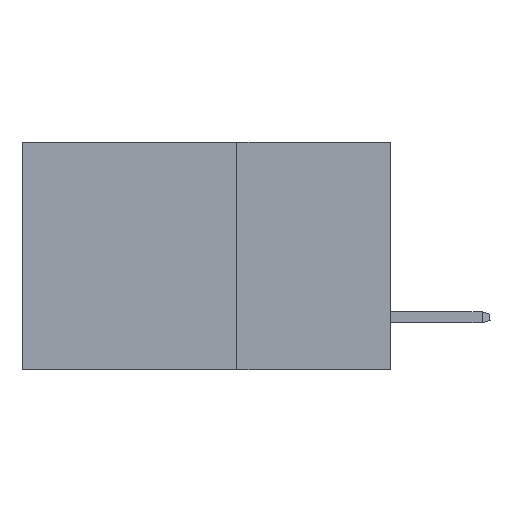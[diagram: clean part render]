
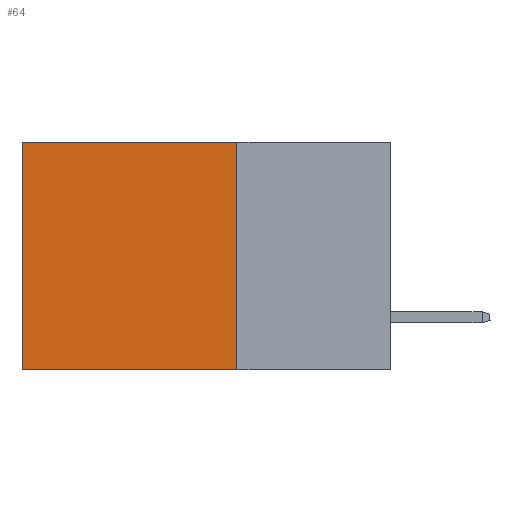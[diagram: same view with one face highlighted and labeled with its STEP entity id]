
A CAD part, left-side view. The second image highlights one B-rep face of the part: STEP entity #64.
In plain terms, the highlighted planar face has unit normal (-1, 0, 0).
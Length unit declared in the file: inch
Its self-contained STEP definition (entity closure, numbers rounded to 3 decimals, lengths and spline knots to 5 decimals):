
#64 = ADVANCED_FACE ( 'NONE', ( #3628 ), #10344, .F. ) ;
#245 = CARTESIAN_POINT ( 'NONE',  ( 0.2875, 0.25, 0. ) ) ;
#1319 = EDGE_CURVE ( 'NONE', #6319, #15988, #18120, .T. ) ;
#1589 = DIRECTION ( 'NONE',  ( 0., 1., 0. ) ) ;
#2468 = CARTESIAN_POINT ( 'NONE',  ( 0.2875, 0.25, -0.37 ) ) ;
#3016 = CARTESIAN_POINT ( 'NONE',  ( 0.2875, 0.6, 0. ) ) ;
#3053 = EDGE_LOOP ( 'NONE', ( #12488, #9216, #9574, #20520 ) ) ;
#3628 = FACE_OUTER_BOUND ( 'NONE', #3053, .T. ) ;
#4110 = VERTEX_POINT ( 'NONE', #13730 ) ;
#4357 = LINE ( 'NONE', #3016, #16062 ) ;
#5113 = DIRECTION ( 'NONE',  ( 0., 1., 0. ) ) ;
#6208 = VERTEX_POINT ( 'NONE', #19198 ) ;
#6319 = VERTEX_POINT ( 'NONE', #245 ) ;
#6855 = LINE ( 'NONE', #15845, #17553 ) ;
#7472 = CARTESIAN_POINT ( 'NONE',  ( 0.2875, 0.25, 0. ) ) ;
#9216 = ORIENTED_EDGE ( 'NONE', *, *, #19005, .F. ) ;
#9574 = ORIENTED_EDGE ( 'NONE', *, *, #1319, .F. ) ;
#10344 = PLANE ( 'NONE',  #15022 ) ;
#11722 = EDGE_CURVE ( 'NONE', #6319, #6208, #13207, .T. ) ;
#12416 = DIRECTION ( 'NONE',  ( 0., 0., -1. ) ) ;
#12488 = ORIENTED_EDGE ( 'NONE', *, *, #20125, .T. ) ;
#13026 = CARTESIAN_POINT ( 'NONE',  ( 0.2875, 0.25, 0. ) ) ;
#13207 = LINE ( 'NONE', #13026, #17962 ) ;
#13730 = CARTESIAN_POINT ( 'NONE',  ( 0.2875, 0.6, -0.37 ) ) ;
#14188 = CARTESIAN_POINT ( 'NONE',  ( 0.2875, 0.25, 0. ) ) ;
#15022 = AXIS2_PLACEMENT_3D ( 'NONE', #7472, #20350, #12416 ) ;
#15845 = CARTESIAN_POINT ( 'NONE',  ( 0.2875, 0.25, -0.37 ) ) ;
#15988 = VERTEX_POINT ( 'NONE', #2468 ) ;
#16062 = VECTOR ( 'NONE', #20322, 39.37008 ) ;
#16129 = VECTOR ( 'NONE', #20327, 39.37008 ) ;
#17553 = VECTOR ( 'NONE', #1589, 39.37008 ) ;
#17962 = VECTOR ( 'NONE', #5113, 39.37008 ) ;
#18120 = LINE ( 'NONE', #14188, #16129 ) ;
#19005 = EDGE_CURVE ( 'NONE', #15988, #4110, #6855, .T. ) ;
#19198 = CARTESIAN_POINT ( 'NONE',  ( 0.2875, 0.6, 0. ) ) ;
#20125 = EDGE_CURVE ( 'NONE', #6208, #4110, #4357, .T. ) ;
#20322 = DIRECTION ( 'NONE',  ( 0., 0., -1. ) ) ;
#20327 = DIRECTION ( 'NONE',  ( 0., 0., -1. ) ) ;
#20350 = DIRECTION ( 'NONE',  ( 1., 0., 0. ) ) ;
#20520 = ORIENTED_EDGE ( 'NONE', *, *, #11722, .T. ) ;
